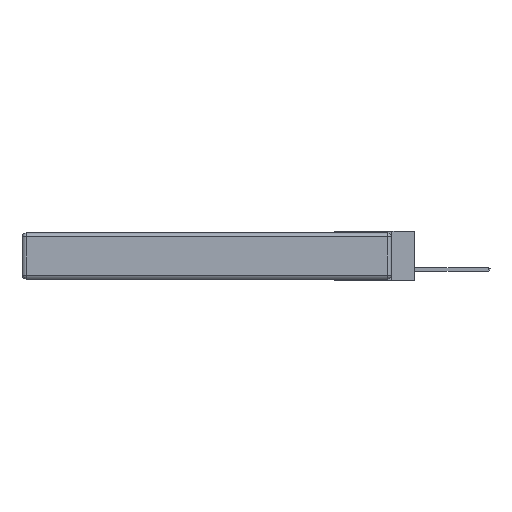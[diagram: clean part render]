
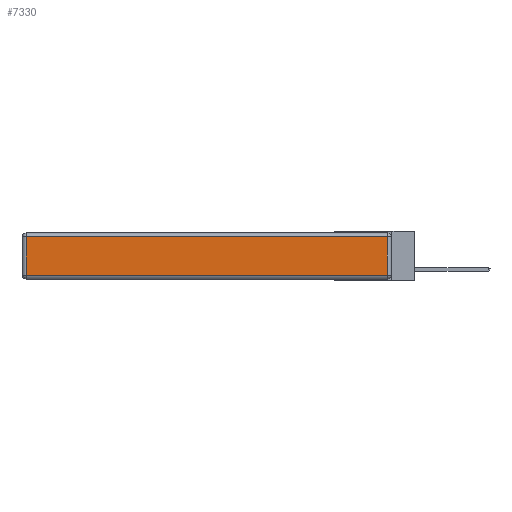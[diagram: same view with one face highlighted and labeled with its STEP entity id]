
A CAD part, left-side view. The second image highlights one B-rep face of the part: STEP entity #7330.
In plain terms, the highlighted planar face has unit normal (-1, 0, 0).
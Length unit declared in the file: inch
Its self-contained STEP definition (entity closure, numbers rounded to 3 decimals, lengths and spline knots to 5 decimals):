
#181 = EDGE_LOOP ( 'NONE', ( #2971, #3603, #6276, #1566 ) ) ;
#886 = VERTEX_POINT ( 'NONE', #4495 ) ;
#921 = DIRECTION ( 'NONE',  ( 0., 0., -1. ) ) ;
#1328 = CARTESIAN_POINT ( 'NONE',  ( 0., 2.72, -0.313 ) ) ;
#1335 = DIRECTION ( 'NONE',  ( 0., -1., 0. ) ) ;
#1566 = ORIENTED_EDGE ( 'NONE', *, *, #10707, .T. ) ;
#1909 = LINE ( 'NONE', #5982, #9898 ) ;
#2413 = CARTESIAN_POINT ( 'NONE',  ( 0., 0.03, -0.343 ) ) ;
#2543 = DIRECTION ( 'NONE',  ( 0., 1., 0. ) ) ;
#2607 = LINE ( 'NONE', #2413, #8536 ) ;
#2971 = ORIENTED_EDGE ( 'NONE', *, *, #11232, .T. ) ;
#3603 = ORIENTED_EDGE ( 'NONE', *, *, #7108, .T. ) ;
#4104 = DIRECTION ( 'NONE',  ( -1., 0., 0. ) ) ;
#4495 = CARTESIAN_POINT ( 'NONE',  ( 0., 0.03, -0.313 ) ) ;
#5982 = CARTESIAN_POINT ( 'NONE',  ( 0., 2.72, -0.343 ) ) ;
#6028 = CARTESIAN_POINT ( 'NONE',  ( 0., 0.03, -0.03 ) ) ;
#6195 = VECTOR ( 'NONE', #1335, 39.37008 ) ;
#6276 = ORIENTED_EDGE ( 'NONE', *, *, #6601, .T. ) ;
#6601 = EDGE_CURVE ( 'NONE', #10693, #8800, #7258, .T. ) ;
#6625 = AXIS2_PLACEMENT_3D ( 'NONE', #12955, #4104, #11301 ) ;
#7108 = EDGE_CURVE ( 'NONE', #886, #10693, #2607, .T. ) ;
#7258 = LINE ( 'NONE', #8625, #8560 ) ;
#7330 = ADVANCED_FACE ( 'NONE', ( #10129 ), #9824, .T. ) ;
#7450 = CARTESIAN_POINT ( 'NONE',  ( 0., 0., -0.313 ) ) ;
#7636 = LINE ( 'NONE', #7450, #6195 ) ;
#8536 = VECTOR ( 'NONE', #12969, 39.37008 ) ;
#8556 = VERTEX_POINT ( 'NONE', #1328 ) ;
#8560 = VECTOR ( 'NONE', #2543, 39.37008 ) ;
#8625 = CARTESIAN_POINT ( 'NONE',  ( 0., 2.75, -0.03 ) ) ;
#8800 = VERTEX_POINT ( 'NONE', #13222 ) ;
#9824 = PLANE ( 'NONE',  #6625 ) ;
#9898 = VECTOR ( 'NONE', #921, 39.37008 ) ;
#10129 = FACE_OUTER_BOUND ( 'NONE', #181, .T. ) ;
#10693 = VERTEX_POINT ( 'NONE', #6028 ) ;
#10707 = EDGE_CURVE ( 'NONE', #8800, #8556, #1909, .T. ) ;
#11232 = EDGE_CURVE ( 'NONE', #8556, #886, #7636, .T. ) ;
#11301 = DIRECTION ( 'NONE',  ( 0., 0., 1. ) ) ;
#12955 = CARTESIAN_POINT ( 'NONE',  ( 0., 0., -0.343 ) ) ;
#12969 = DIRECTION ( 'NONE',  ( 0., 0., 1. ) ) ;
#13222 = CARTESIAN_POINT ( 'NONE',  ( 0., 2.72, -0.03 ) ) ;
